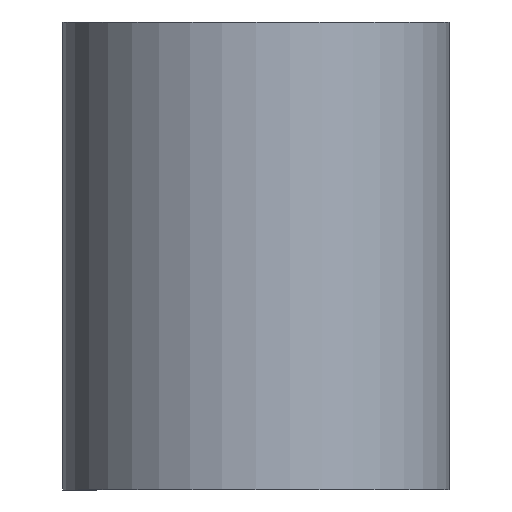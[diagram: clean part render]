
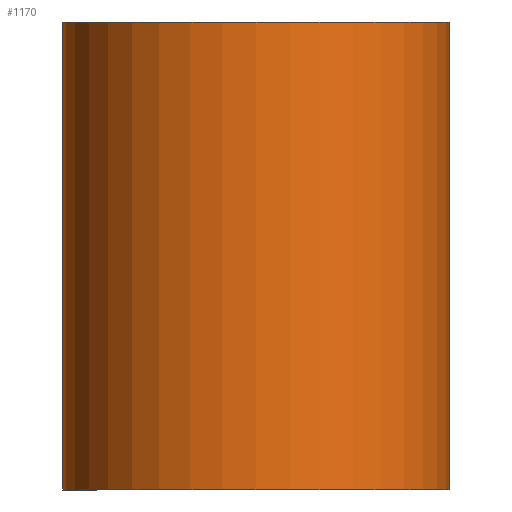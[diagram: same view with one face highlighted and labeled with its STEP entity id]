
A CAD part, front view. The second image highlights one B-rep face of the part: STEP entity #1170.
In plain terms, the highlighted cylindrical face has radius 18.567 mm (diameter 37.133 mm), a partial arc.
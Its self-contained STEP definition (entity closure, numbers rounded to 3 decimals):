
#21 = AXIS2_PLACEMENT_3D ( 'NONE', #1417, #1161, #306 ) ;
#50 = VERTEX_POINT ( 'NONE', #730 ) ;
#77 = VECTOR ( 'NONE', #152, 1000. ) ;
#108 = CARTESIAN_POINT ( 'NONE',  ( -190.165, -88.078, 22.512 ) ) ;
#143 = VERTEX_POINT ( 'NONE', #423 ) ;
#152 = DIRECTION ( 'NONE',  ( 0., 0., 1. ) ) ;
#200 = EDGE_CURVE ( 'NONE', #1275, #1004, #1354, .T. ) ;
#306 = DIRECTION ( 'NONE',  ( -1., 0., 0. ) ) ;
#397 = DIRECTION ( 'NONE',  ( 0., 0., 1. ) ) ;
#423 = CARTESIAN_POINT ( 'NONE',  ( -171.598, -88.078, -22.488 ) ) ;
#451 = DIRECTION ( 'NONE',  ( -1., 0., 0. ) ) ;
#510 = ORIENTED_EDGE ( 'NONE', *, *, #878, .T. ) ;
#573 = DIRECTION ( 'NONE',  ( 0., 0., 1. ) ) ;
#592 = ORIENTED_EDGE ( 'NONE', *, *, #1459, .T. ) ;
#622 = DIRECTION ( 'NONE',  ( 0., 0., 1. ) ) ;
#631 = CARTESIAN_POINT ( 'NONE',  ( -208.731, -88.078, -22.488 ) ) ;
#730 = CARTESIAN_POINT ( 'NONE',  ( -171.598, -88.078, 22.512 ) ) ;
#758 = CYLINDRICAL_SURFACE ( 'NONE', #1324, 18.567 ) ;
#876 = CARTESIAN_POINT ( 'NONE',  ( -208.731, -88.078, -22.488 ) ) ;
#878 = EDGE_CURVE ( 'NONE', #1275, #143, #1381, .T. ) ;
#928 = ORIENTED_EDGE ( 'NONE', *, *, #200, .F. ) ;
#976 = DIRECTION ( 'NONE',  ( 1., 0., 0. ) ) ;
#1004 = VERTEX_POINT ( 'NONE', #1422 ) ;
#1005 = VECTOR ( 'NONE', #622, 1000. ) ;
#1156 = EDGE_CURVE ( 'NONE', #1004, #50, #1484, .T. ) ;
#1161 = DIRECTION ( 'NONE',  ( 0., 0., 1. ) ) ;
#1170 = ADVANCED_FACE ( 'NONE', ( #1355 ), #758, .T. ) ;
#1197 = AXIS2_PLACEMENT_3D ( 'NONE', #108, #573, #451 ) ;
#1275 = VERTEX_POINT ( 'NONE', #876 ) ;
#1324 = AXIS2_PLACEMENT_3D ( 'NONE', #1577, #397, #976 ) ;
#1354 = LINE ( 'NONE', #631, #1005 ) ;
#1355 = FACE_OUTER_BOUND ( 'NONE', #1485, .T. ) ;
#1379 = LINE ( 'NONE', #1528, #77 ) ;
#1381 = CIRCLE ( 'NONE', #21, 18.567 ) ;
#1417 = CARTESIAN_POINT ( 'NONE',  ( -190.165, -88.078, -22.488 ) ) ;
#1422 = CARTESIAN_POINT ( 'NONE',  ( -208.731, -88.078, 22.512 ) ) ;
#1459 = EDGE_CURVE ( 'NONE', #143, #50, #1379, .T. ) ;
#1484 = CIRCLE ( 'NONE', #1197, 18.567 ) ;
#1485 = EDGE_LOOP ( 'NONE', ( #1488, #928, #510, #592 ) ) ;
#1488 = ORIENTED_EDGE ( 'NONE', *, *, #1156, .F. ) ;
#1528 = CARTESIAN_POINT ( 'NONE',  ( -171.598, -88.078, -22.488 ) ) ;
#1577 = CARTESIAN_POINT ( 'NONE',  ( -190.165, -88.078, -22.488 ) ) ;
